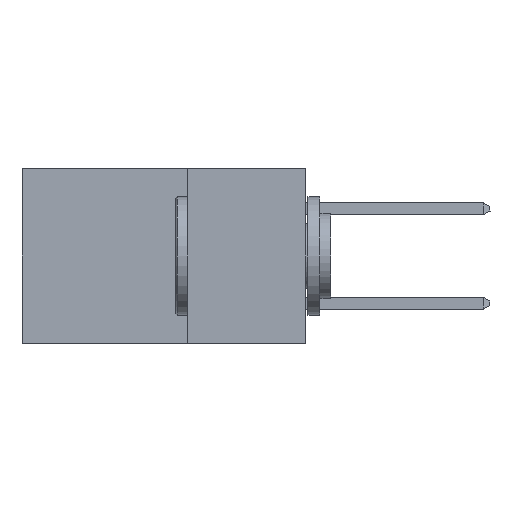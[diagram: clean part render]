
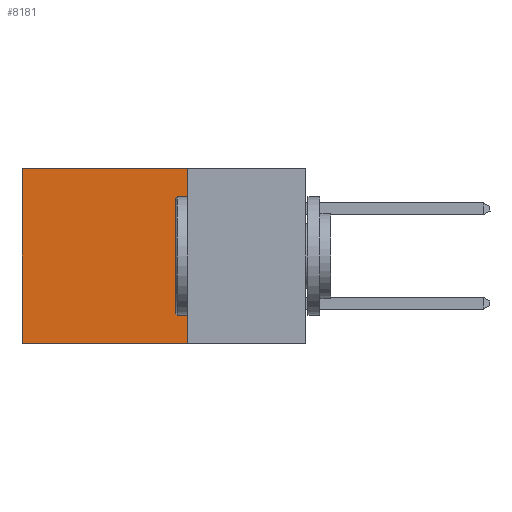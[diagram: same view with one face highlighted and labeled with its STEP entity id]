
A CAD part, left-side view. The second image highlights one B-rep face of the part: STEP entity #8181.
In plain terms, the highlighted planar face has unit normal (-1, 0, 0).
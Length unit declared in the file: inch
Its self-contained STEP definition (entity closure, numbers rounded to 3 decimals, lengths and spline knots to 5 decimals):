
#185 = CARTESIAN_POINT ( 'NONE',  ( 0.298, 0.6, 0. ) ) ;
#315 = VERTEX_POINT ( 'NONE', #1388 ) ;
#524 = DIRECTION ( 'NONE',  ( 1., 0., 0. ) ) ;
#775 = DIRECTION ( 'NONE',  ( 0., 1., 0. ) ) ;
#822 = VERTEX_POINT ( 'NONE', #8081 ) ;
#1171 = ORIENTED_EDGE ( 'NONE', *, *, #10670, .T. ) ;
#1370 = LINE ( 'NONE', #13348, #14732 ) ;
#1388 = CARTESIAN_POINT ( 'NONE',  ( 0.298, 0.6, -0.37 ) ) ;
#1646 = CARTESIAN_POINT ( 'NONE',  ( 0.298, 0.25, 0. ) ) ;
#1744 = VERTEX_POINT ( 'NONE', #4128 ) ;
#2083 = EDGE_LOOP ( 'NONE', ( #7837, #3868, #6461, #1171 ) ) ;
#2210 = VERTEX_POINT ( 'NONE', #8863 ) ;
#2501 = CARTESIAN_POINT ( 'NONE',  ( 0.298, 0.25, 0. ) ) ;
#2627 = EDGE_CURVE ( 'NONE', #2210, #315, #4685, .T. ) ;
#3438 = VECTOR ( 'NONE', #775, 39.37008 ) ;
#3614 = DIRECTION ( 'NONE',  ( 0., 0., -1. ) ) ;
#3700 = DIRECTION ( 'NONE',  ( 0., 1., 0. ) ) ;
#3868 = ORIENTED_EDGE ( 'NONE', *, *, #7714, .F. ) ;
#4128 = CARTESIAN_POINT ( 'NONE',  ( 0.298, 0.25, -0.37 ) ) ;
#4685 = LINE ( 'NONE', #185, #14344 ) ;
#6332 = PLANE ( 'NONE',  #7467 ) ;
#6377 = CARTESIAN_POINT ( 'NONE',  ( 0.298, 0.25, -0.37 ) ) ;
#6461 = ORIENTED_EDGE ( 'NONE', *, *, #8282, .F. ) ;
#7467 = AXIS2_PLACEMENT_3D ( 'NONE', #1646, #524, #14338 ) ;
#7714 = EDGE_CURVE ( 'NONE', #1744, #315, #12366, .T. ) ;
#7837 = ORIENTED_EDGE ( 'NONE', *, *, #2627, .T. ) ;
#8081 = CARTESIAN_POINT ( 'NONE',  ( 0.298, 0.25, 0. ) ) ;
#8181 = ADVANCED_FACE ( 'NONE', ( #11486 ), #6332, .F. ) ;
#8282 = EDGE_CURVE ( 'NONE', #822, #1744, #1370, .T. ) ;
#8863 = CARTESIAN_POINT ( 'NONE',  ( 0.298, 0.6, 0. ) ) ;
#9198 = LINE ( 'NONE', #2501, #12130 ) ;
#10670 = EDGE_CURVE ( 'NONE', #822, #2210, #9198, .T. ) ;
#11068 = DIRECTION ( 'NONE',  ( 0., 0., -1. ) ) ;
#11486 = FACE_OUTER_BOUND ( 'NONE', #2083, .T. ) ;
#12130 = VECTOR ( 'NONE', #3700, 39.37008 ) ;
#12366 = LINE ( 'NONE', #6377, #3438 ) ;
#13348 = CARTESIAN_POINT ( 'NONE',  ( 0.298, 0.25, 0. ) ) ;
#14338 = DIRECTION ( 'NONE',  ( 0., 0., -1. ) ) ;
#14344 = VECTOR ( 'NONE', #3614, 39.37008 ) ;
#14732 = VECTOR ( 'NONE', #11068, 39.37008 ) ;
